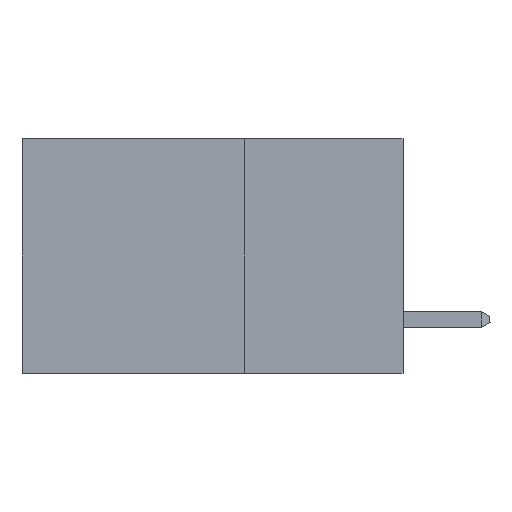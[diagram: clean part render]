
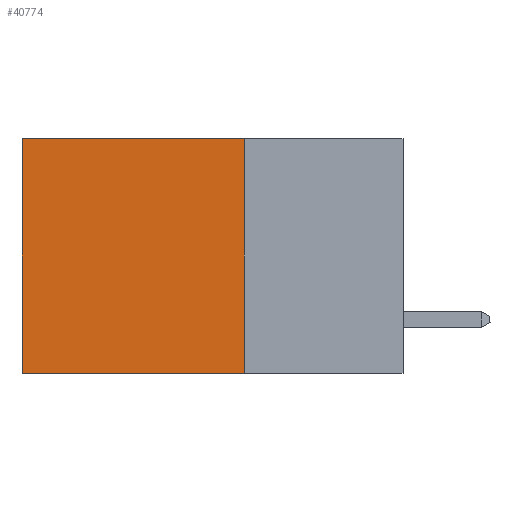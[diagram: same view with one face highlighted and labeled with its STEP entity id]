
A CAD part, left-side view. The second image highlights one B-rep face of the part: STEP entity #40774.
In plain terms, the highlighted planar face has unit normal (-1, 0, 0).
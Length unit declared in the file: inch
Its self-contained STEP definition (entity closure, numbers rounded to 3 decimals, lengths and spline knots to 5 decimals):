
#327 = VERTEX_POINT ( 'NONE', #39702 ) ;
#957 = AXIS2_PLACEMENT_3D ( 'NONE', #31060, #41993, #16962 ) ;
#6779 = ORIENTED_EDGE ( 'NONE', *, *, #39291, .T. ) ;
#8677 = LINE ( 'NONE', #19096, #12557 ) ;
#9532 = CARTESIAN_POINT ( 'NONE',  ( 0.2875, 0.25, 0. ) ) ;
#10500 = ORIENTED_EDGE ( 'NONE', *, *, #29070, .F. ) ;
#11284 = EDGE_CURVE ( 'NONE', #19426, #44746, #20675, .T. ) ;
#12557 = VECTOR ( 'NONE', #26229, 39.37008 ) ;
#16962 = DIRECTION ( 'NONE',  ( 0., 0., -1. ) ) ;
#17641 = DIRECTION ( 'NONE',  ( 0., 0., -1. ) ) ;
#18383 = VECTOR ( 'NONE', #17641, 39.37008 ) ;
#19096 = CARTESIAN_POINT ( 'NONE',  ( 0.2875, 0.25, 0. ) ) ;
#19426 = VERTEX_POINT ( 'NONE', #27147 ) ;
#19958 = DIRECTION ( 'NONE',  ( 0., 1., 0. ) ) ;
#19995 = FACE_OUTER_BOUND ( 'NONE', #31020, .T. ) ;
#20675 = LINE ( 'NONE', #9532, #38376 ) ;
#21158 = CARTESIAN_POINT ( 'NONE',  ( 0.2875, 0.6, -0.37 ) ) ;
#23197 = VECTOR ( 'NONE', #19958, 39.37008 ) ;
#24307 = LINE ( 'NONE', #37400, #23197 ) ;
#24641 = CARTESIAN_POINT ( 'NONE',  ( 0.2875, 0.25, -0.37 ) ) ;
#26229 = DIRECTION ( 'NONE',  ( 0., 1., 0. ) ) ;
#27147 = CARTESIAN_POINT ( 'NONE',  ( 0.2875, 0.25, 0. ) ) ;
#27870 = LINE ( 'NONE', #31125, #18383 ) ;
#29070 = EDGE_CURVE ( 'NONE', #44746, #29431, #24307, .T. ) ;
#29431 = VERTEX_POINT ( 'NONE', #21158 ) ;
#29696 = EDGE_CURVE ( 'NONE', #19426, #327, #8677, .T. ) ;
#30077 = ORIENTED_EDGE ( 'NONE', *, *, #29696, .T. ) ;
#31020 = EDGE_LOOP ( 'NONE', ( #6779, #10500, #34784, #30077 ) ) ;
#31060 = CARTESIAN_POINT ( 'NONE',  ( 0.2875, 0.25, 0. ) ) ;
#31125 = CARTESIAN_POINT ( 'NONE',  ( 0.2875, 0.6, 0. ) ) ;
#34784 = ORIENTED_EDGE ( 'NONE', *, *, #11284, .F. ) ;
#37400 = CARTESIAN_POINT ( 'NONE',  ( 0.2875, 0.25, -0.37 ) ) ;
#38376 = VECTOR ( 'NONE', #40964, 39.37008 ) ;
#39291 = EDGE_CURVE ( 'NONE', #327, #29431, #27870, .T. ) ;
#39702 = CARTESIAN_POINT ( 'NONE',  ( 0.2875, 0.6, 0. ) ) ;
#40774 = ADVANCED_FACE ( 'NONE', ( #19995 ), #45703, .F. ) ;
#40964 = DIRECTION ( 'NONE',  ( 0., 0., -1. ) ) ;
#41993 = DIRECTION ( 'NONE',  ( 1., 0., 0. ) ) ;
#44746 = VERTEX_POINT ( 'NONE', #24641 ) ;
#45703 = PLANE ( 'NONE',  #957 ) ;
